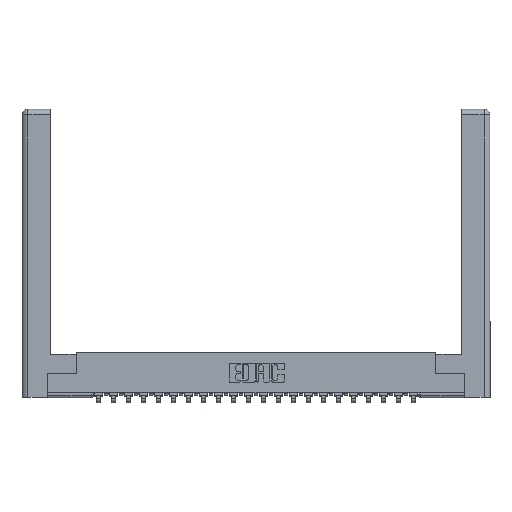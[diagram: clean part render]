
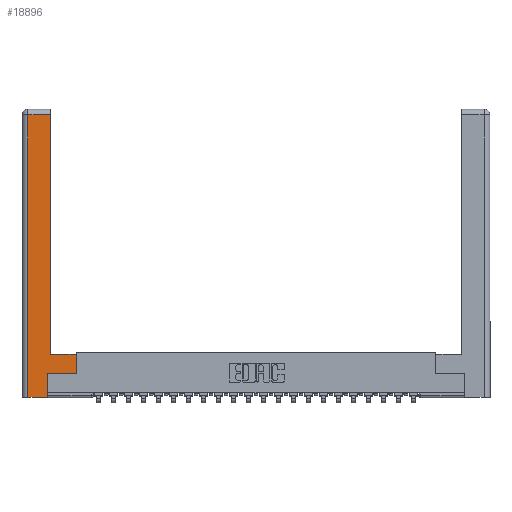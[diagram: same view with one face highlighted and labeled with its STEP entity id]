
A CAD part, top view. The second image highlights one B-rep face of the part: STEP entity #18896.
In plain terms, the highlighted planar face has unit normal (0, 0, 1).
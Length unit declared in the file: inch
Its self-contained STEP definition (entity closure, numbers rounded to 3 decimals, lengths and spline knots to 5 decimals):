
#1052 = VERTEX_POINT ( 'NONE', #20932 ) ;
#1181 = ORIENTED_EDGE ( 'NONE', *, *, #10799, .T. ) ;
#1758 = EDGE_CURVE ( 'NONE', #16964, #21270, #14705, .T. ) ;
#1848 = ORIENTED_EDGE ( 'NONE', *, *, #6364, .T. ) ;
#2197 = EDGE_CURVE ( 'NONE', #18301, #13965, #6148, .T. ) ;
#3069 = DIRECTION ( 'NONE',  ( -1., 0., 0. ) ) ;
#3688 = EDGE_CURVE ( 'NONE', #13965, #16964, #21461, .T. ) ;
#3957 = CARTESIAN_POINT ( 'NONE',  ( 0.265, 0.245, 0. ) ) ;
#3962 = DIRECTION ( 'NONE',  ( 0., -1., 0. ) ) ;
#4677 = VERTEX_POINT ( 'NONE', #23179 ) ;
#6024 = DIRECTION ( 'NONE',  ( 1., 0., 0. ) ) ;
#6148 = LINE ( 'NONE', #19967, #10839 ) ;
#6335 = ORIENTED_EDGE ( 'NONE', *, *, #3688, .T. ) ;
#6364 = EDGE_CURVE ( 'NONE', #4677, #23681, #19382, .T. ) ;
#6706 = VERTEX_POINT ( 'NONE', #23253 ) ;
#7321 = ORIENTED_EDGE ( 'NONE', *, *, #1758, .T. ) ;
#8267 = EDGE_CURVE ( 'NONE', #23681, #6706, #16511, .T. ) ;
#8315 = CARTESIAN_POINT ( 'NONE',  ( 0.295, 3., 0. ) ) ;
#9627 = VECTOR ( 'NONE', #21501, 39.37008 ) ;
#10320 = VECTOR ( 'NONE', #3962, 39.37008 ) ;
#10755 = VECTOR ( 'NONE', #20106, 39.37008 ) ;
#10799 = EDGE_CURVE ( 'NONE', #1052, #18301, #15573, .T. ) ;
#10826 = DIRECTION ( 'NONE',  ( 0., 0., -1. ) ) ;
#10839 = VECTOR ( 'NONE', #17738, 39.37008 ) ;
#10923 = CARTESIAN_POINT ( 'NONE',  ( 0.565, 0.45, 0. ) ) ;
#12241 = CARTESIAN_POINT ( 'NONE',  ( 0.565, 0.245, 0. ) ) ;
#12709 = PLANE ( 'NONE',  #13139 ) ;
#12761 = CARTESIAN_POINT ( 'NONE',  ( 0.295, 2.94, 0. ) ) ;
#13139 = AXIS2_PLACEMENT_3D ( 'NONE', #20381, #10826, #18509 ) ;
#13965 = VERTEX_POINT ( 'NONE', #3957 ) ;
#14277 = DIRECTION ( 'NONE',  ( 1., 0., 0. ) ) ;
#14320 = LINE ( 'NONE', #21990, #10755 ) ;
#14705 = LINE ( 'NONE', #10923, #15216 ) ;
#15216 = VECTOR ( 'NONE', #24263, 39.37008 ) ;
#15573 = LINE ( 'NONE', #23250, #16718 ) ;
#16106 = VECTOR ( 'NONE', #3069, 39.37008 ) ;
#16453 = CARTESIAN_POINT ( 'NONE',  ( 0.565, 0.45, 0. ) ) ;
#16511 = LINE ( 'NONE', #20528, #16106 ) ;
#16718 = VECTOR ( 'NONE', #6024, 39.37008 ) ;
#16964 = VERTEX_POINT ( 'NONE', #12241 ) ;
#17687 = CARTESIAN_POINT ( 'NONE',  ( 0.265, 0., 0. ) ) ;
#17713 = CARTESIAN_POINT ( 'NONE',  ( 0.565, 0.245, 0. ) ) ;
#17738 = DIRECTION ( 'NONE',  ( 0., 1., 0. ) ) ;
#18239 = ORIENTED_EDGE ( 'NONE', *, *, #8267, .T. ) ;
#18301 = VERTEX_POINT ( 'NONE', #17687 ) ;
#18509 = DIRECTION ( 'NONE',  ( -1., 0., 0. ) ) ;
#18589 = EDGE_CURVE ( 'NONE', #6706, #1052, #20795, .T. ) ;
#18896 = ADVANCED_FACE ( 'NONE', ( #24160 ), #12709, .F. ) ;
#19049 = ORIENTED_EDGE ( 'NONE', *, *, #22453, .T. ) ;
#19382 = LINE ( 'NONE', #8315, #9627 ) ;
#19967 = CARTESIAN_POINT ( 'NONE',  ( 0.265, 0.245, 0. ) ) ;
#20106 = DIRECTION ( 'NONE',  ( -1., 0., 0. ) ) ;
#20302 = ORIENTED_EDGE ( 'NONE', *, *, #18589, .T. ) ;
#20381 = CARTESIAN_POINT ( 'NONE',  ( 0., 0., 0. ) ) ;
#20528 = CARTESIAN_POINT ( 'NONE',  ( 0.0615, 2.94, 0. ) ) ;
#20664 = CARTESIAN_POINT ( 'NONE',  ( 0.0615, 0., 0. ) ) ;
#20795 = LINE ( 'NONE', #20664, #10320 ) ;
#20932 = CARTESIAN_POINT ( 'NONE',  ( 0.0615, 0., 0. ) ) ;
#21270 = VERTEX_POINT ( 'NONE', #16453 ) ;
#21461 = LINE ( 'NONE', #17713, #22506 ) ;
#21501 = DIRECTION ( 'NONE',  ( 0., 1., 0. ) ) ;
#21990 = CARTESIAN_POINT ( 'NONE',  ( 0.295, 0.45, 0. ) ) ;
#22453 = EDGE_CURVE ( 'NONE', #21270, #4677, #14320, .T. ) ;
#22506 = VECTOR ( 'NONE', #14277, 39.37008 ) ;
#23055 = ORIENTED_EDGE ( 'NONE', *, *, #2197, .T. ) ;
#23179 = CARTESIAN_POINT ( 'NONE',  ( 0.295, 0.45, 0. ) ) ;
#23250 = CARTESIAN_POINT ( 'NONE',  ( 0.265, 0., 0. ) ) ;
#23253 = CARTESIAN_POINT ( 'NONE',  ( 0.0615, 2.94, 0. ) ) ;
#23681 = VERTEX_POINT ( 'NONE', #12761 ) ;
#24117 = EDGE_LOOP ( 'NONE', ( #1848, #18239, #20302, #1181, #23055, #6335, #7321, #19049 ) ) ;
#24160 = FACE_OUTER_BOUND ( 'NONE', #24117, .T. ) ;
#24263 = DIRECTION ( 'NONE',  ( 0., 1., 0. ) ) ;
